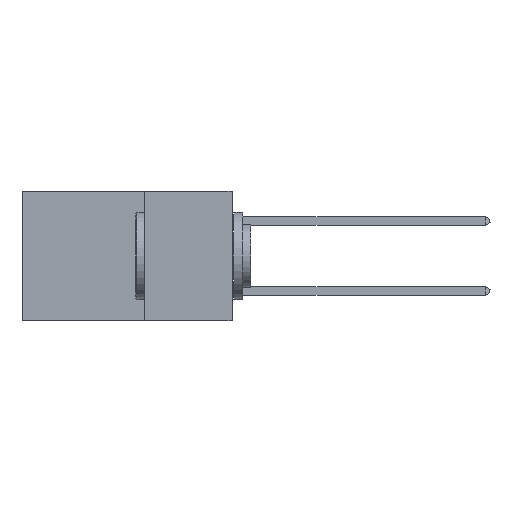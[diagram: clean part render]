
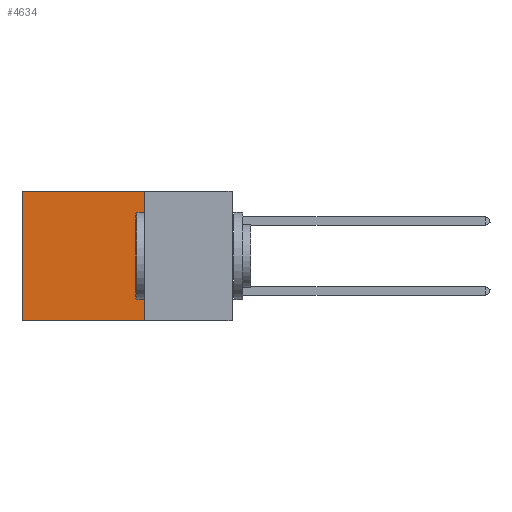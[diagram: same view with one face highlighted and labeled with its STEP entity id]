
A CAD part, left-side view. The second image highlights one B-rep face of the part: STEP entity #4634.
In plain terms, the highlighted planar face has unit normal (-1, 0, 0).
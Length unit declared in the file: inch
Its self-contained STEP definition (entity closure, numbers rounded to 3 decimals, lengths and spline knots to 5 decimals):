
#1719 = PLANE ( 'NONE',  #18259 ) ;
#2143 = DIRECTION ( 'NONE',  ( 0., 1., 0. ) ) ;
#2775 = DIRECTION ( 'NONE',  ( 0., 0., -1. ) ) ;
#2780 = EDGE_CURVE ( 'NONE', #30494, #6862, #8897, .T. ) ;
#4634 = ADVANCED_FACE ( 'NONE', ( #14074 ), #1719, .F. ) ;
#5327 = EDGE_CURVE ( 'NONE', #14880, #30494, #15148, .T. ) ;
#6684 = CARTESIAN_POINT ( 'NONE',  ( 0.2875, 0.25, 0. ) ) ;
#6862 = VERTEX_POINT ( 'NONE', #17857 ) ;
#7283 = VECTOR ( 'NONE', #2775, 39.37008 ) ;
#7770 = VERTEX_POINT ( 'NONE', #30854 ) ;
#7908 = CARTESIAN_POINT ( 'NONE',  ( 0.2875, 0.25, 0. ) ) ;
#8158 = VECTOR ( 'NONE', #2143, 39.37008 ) ;
#8897 = LINE ( 'NONE', #26060, #8158 ) ;
#9119 = DIRECTION ( 'NONE',  ( 0., 0., -1. ) ) ;
#10018 = EDGE_CURVE ( 'NONE', #7770, #6862, #11810, .T. ) ;
#11810 = LINE ( 'NONE', #13096, #23714 ) ;
#12076 = DIRECTION ( 'NONE',  ( 0., 1., 0. ) ) ;
#12323 = CARTESIAN_POINT ( 'NONE',  ( 0.2875, 0.25, 0. ) ) ;
#13096 = CARTESIAN_POINT ( 'NONE',  ( 0.2875, 0.6, 0. ) ) ;
#13931 = EDGE_LOOP ( 'NONE', ( #14176, #21056, #26924, #25845 ) ) ;
#14074 = FACE_OUTER_BOUND ( 'NONE', #13931, .T. ) ;
#14176 = ORIENTED_EDGE ( 'NONE', *, *, #10018, .T. ) ;
#14880 = VERTEX_POINT ( 'NONE', #7908 ) ;
#15148 = LINE ( 'NONE', #12323, #7283 ) ;
#17857 = CARTESIAN_POINT ( 'NONE',  ( 0.2875, 0.6, -0.37 ) ) ;
#17877 = DIRECTION ( 'NONE',  ( 0., 0., -1. ) ) ;
#18259 = AXIS2_PLACEMENT_3D ( 'NONE', #6684, #23382, #9119 ) ;
#18356 = VECTOR ( 'NONE', #12076, 39.37008 ) ;
#21056 = ORIENTED_EDGE ( 'NONE', *, *, #2780, .F. ) ;
#21613 = EDGE_CURVE ( 'NONE', #14880, #7770, #25406, .T. ) ;
#23257 = CARTESIAN_POINT ( 'NONE',  ( 0.2875, 0.25, -0.37 ) ) ;
#23382 = DIRECTION ( 'NONE',  ( 1., 0., 0. ) ) ;
#23714 = VECTOR ( 'NONE', #17877, 39.37008 ) ;
#24030 = CARTESIAN_POINT ( 'NONE',  ( 0.2875, 0.25, 0. ) ) ;
#25406 = LINE ( 'NONE', #24030, #18356 ) ;
#25845 = ORIENTED_EDGE ( 'NONE', *, *, #21613, .T. ) ;
#26060 = CARTESIAN_POINT ( 'NONE',  ( 0.2875, 0.25, -0.37 ) ) ;
#26924 = ORIENTED_EDGE ( 'NONE', *, *, #5327, .F. ) ;
#30494 = VERTEX_POINT ( 'NONE', #23257 ) ;
#30854 = CARTESIAN_POINT ( 'NONE',  ( 0.2875, 0.6, 0. ) ) ;
